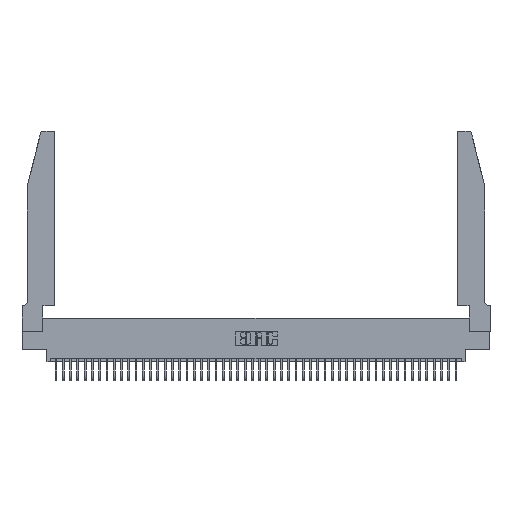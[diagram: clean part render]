
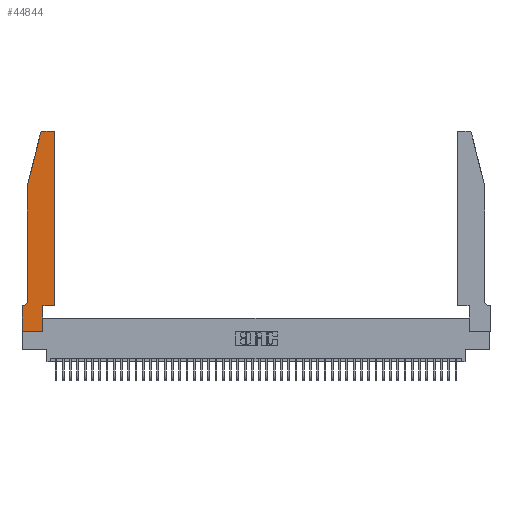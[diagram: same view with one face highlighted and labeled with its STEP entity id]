
A CAD part, top view. The second image highlights one B-rep face of the part: STEP entity #44844.
In plain terms, the highlighted planar face has unit normal (0, 0, 1).
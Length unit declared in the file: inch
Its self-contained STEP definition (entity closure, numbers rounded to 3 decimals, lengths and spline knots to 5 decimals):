
#1173 = CARTESIAN_POINT ( 'NONE',  ( 0.284, 2.75, 0.37 ) ) ;
#1705 = DIRECTION ( 'NONE',  ( 0., 0., -1. ) ) ;
#1728 = LINE ( 'NONE', #22792, #20487 ) ;
#2215 = DIRECTION ( 'NONE',  ( 0., 0., 1. ) ) ;
#2640 = ORIENTED_EDGE ( 'NONE', *, *, #30692, .T. ) ;
#3220 = DIRECTION ( 'NONE',  ( 0., 0., 1. ) ) ;
#3641 = AXIS2_PLACEMENT_3D ( 'NONE', #38031, #17236, #41556 ) ;
#4060 = ORIENTED_EDGE ( 'NONE', *, *, #23401, .T. ) ;
#4493 = ORIENTED_EDGE ( 'NONE', *, *, #15416, .T. ) ;
#4783 = CARTESIAN_POINT ( 'NONE',  ( 0.4205, 2.75, 0.37 ) ) ;
#5003 = VERTEX_POINT ( 'NONE', #37619 ) ;
#5460 = ORIENTED_EDGE ( 'NONE', *, *, #25876, .T. ) ;
#5517 = VERTEX_POINT ( 'NONE', #40341 ) ;
#5669 = ORIENTED_EDGE ( 'NONE', *, *, #30550, .T. ) ;
#6567 = DIRECTION ( 'NONE',  ( 0., -1., 0. ) ) ;
#6885 = EDGE_CURVE ( 'NONE', #39314, #39342, #33045, .T. ) ;
#7186 = CARTESIAN_POINT ( 'NONE',  ( 0.4505, 0.35, 0.37 ) ) ;
#7637 = VECTOR ( 'NONE', #6567, 39.37008 ) ;
#7947 = CARTESIAN_POINT ( 'NONE',  ( 0.0755, 0.35, 0.37 ) ) ;
#8311 = CIRCLE ( 'NONE', #44895, 0.03 ) ;
#8340 = VECTOR ( 'NONE', #38804, 39.37008 ) ;
#8362 = EDGE_CURVE ( 'NONE', #38802, #43409, #1728, .T. ) ;
#8693 = DIRECTION ( 'NONE',  ( -0.239, -0.971, 0. ) ) ;
#9033 = CARTESIAN_POINT ( 'NONE',  ( 0., 0.35, 0.37 ) ) ;
#9128 = VERTEX_POINT ( 'NONE', #20470 ) ;
#10287 = CIRCLE ( 'NONE', #3641, 0.03 ) ;
#10928 = CARTESIAN_POINT ( 'NONE',  ( 0.25487, 2.72718, 0.37 ) ) ;
#13617 = AXIS2_PLACEMENT_3D ( 'NONE', #33557, #2215, #26706 ) ;
#14084 = DIRECTION ( 'NONE',  ( 0., 1., 0. ) ) ;
#14966 = CARTESIAN_POINT ( 'NONE',  ( 0.0755, 2., 0.37 ) ) ;
#15416 = EDGE_CURVE ( 'NONE', #9128, #39314, #26887, .T. ) ;
#16180 = ORIENTED_EDGE ( 'NONE', *, *, #40834, .T. ) ;
#16627 = DIRECTION ( 'NONE',  ( -1., 0., 0. ) ) ;
#16882 = ORIENTED_EDGE ( 'NONE', *, *, #43784, .T. ) ;
#17236 = DIRECTION ( 'NONE',  ( 0., 0., 1. ) ) ;
#17279 = FACE_OUTER_BOUND ( 'NONE', #21320, .T. ) ;
#19246 = VECTOR ( 'NONE', #42854, 39.37008 ) ;
#20470 = CARTESIAN_POINT ( 'NONE',  ( 0.2865, 0.35, 0.37 ) ) ;
#20487 = VECTOR ( 'NONE', #8693, 39.37008 ) ;
#20929 = ORIENTED_EDGE ( 'NONE', *, *, #38671, .T. ) ;
#21320 = EDGE_LOOP ( 'NONE', ( #4060, #20929, #37957, #5460, #22367, #42710, #16882, #16180, #5669, #4493, #29392, #2640 ) ) ;
#21464 = LINE ( 'NONE', #7947, #19246 ) ;
#22047 = VECTOR ( 'NONE', #44120, 39.37008 ) ;
#22367 = ORIENTED_EDGE ( 'NONE', *, *, #32344, .T. ) ;
#22773 = CARTESIAN_POINT ( 'NONE',  ( 0.0055, 0.42, 0.37 ) ) ;
#22792 = CARTESIAN_POINT ( 'NONE',  ( 0.0755, 2., 0.37 ) ) ;
#23273 = PLANE ( 'NONE',  #13617 ) ;
#23401 = EDGE_CURVE ( 'NONE', #28050, #35162, #42786, .T. ) ;
#23751 = VECTOR ( 'NONE', #29623, 39.37008 ) ;
#24238 = CARTESIAN_POINT ( 'NONE',  ( 0.4205, 2.72, 0.37 ) ) ;
#25876 = EDGE_CURVE ( 'NONE', #43409, #5003, #31627, .T. ) ;
#26091 = CARTESIAN_POINT ( 'NONE',  ( 0.0755, 2., 0.37 ) ) ;
#26190 = DIRECTION ( 'NONE',  ( -1., 0., 0. ) ) ;
#26706 = DIRECTION ( 'NONE',  ( 1., 0., 0. ) ) ;
#26887 = LINE ( 'NONE', #28304, #8340 ) ;
#27705 = DIRECTION ( 'NONE',  ( 1., 0., 0. ) ) ;
#28050 = VERTEX_POINT ( 'NONE', #4783 ) ;
#28246 = CARTESIAN_POINT ( 'NONE',  ( 0.4505, 2.72, 0.37 ) ) ;
#28304 = CARTESIAN_POINT ( 'NONE',  ( 0.4505, 0.35, 0.37 ) ) ;
#29392 = ORIENTED_EDGE ( 'NONE', *, *, #6885, .T. ) ;
#29623 = DIRECTION ( 'NONE',  ( 1., 0., 0. ) ) ;
#30550 = EDGE_CURVE ( 'NONE', #5517, #9128, #40528, .T. ) ;
#30692 = EDGE_CURVE ( 'NONE', #39342, #28050, #8311, .T. ) ;
#31295 = AXIS2_PLACEMENT_3D ( 'NONE', #22773, #1705, #26190 ) ;
#31627 = LINE ( 'NONE', #26091, #39801 ) ;
#32344 = EDGE_CURVE ( 'NONE', #5003, #33185, #34839, .T. ) ;
#32946 = LINE ( 'NONE', #43610, #23751 ) ;
#33045 = LINE ( 'NONE', #38526, #42332 ) ;
#33185 = VERTEX_POINT ( 'NONE', #38495 ) ;
#33557 = CARTESIAN_POINT ( 'NONE',  ( 0., 0.35, 0.37 ) ) ;
#34577 = VECTOR ( 'NONE', #16627, 39.37008 ) ;
#34839 = CIRCLE ( 'NONE', #31295, 0.07 ) ;
#35162 = VERTEX_POINT ( 'NONE', #1173 ) ;
#35440 = LINE ( 'NONE', #44792, #7637 ) ;
#36590 = DIRECTION ( 'NONE',  ( 0., -1., 0. ) ) ;
#37155 = CARTESIAN_POINT ( 'NONE',  ( 0.2865, 0.35, 0.37 ) ) ;
#37302 = VERTEX_POINT ( 'NONE', #9033 ) ;
#37619 = CARTESIAN_POINT ( 'NONE',  ( 0.0755, 0.42, 0.37 ) ) ;
#37620 = VERTEX_POINT ( 'NONE', #42075 ) ;
#37957 = ORIENTED_EDGE ( 'NONE', *, *, #8362, .T. ) ;
#38031 = CARTESIAN_POINT ( 'NONE',  ( 0.284, 2.72, 0.37 ) ) ;
#38495 = CARTESIAN_POINT ( 'NONE',  ( 0.0055, 0.35, 0.37 ) ) ;
#38526 = CARTESIAN_POINT ( 'NONE',  ( 0.4505, 0.35, 0.37 ) ) ;
#38671 = EDGE_CURVE ( 'NONE', #35162, #38802, #10287, .T. ) ;
#38802 = VERTEX_POINT ( 'NONE', #10928 ) ;
#38804 = DIRECTION ( 'NONE',  ( 1., 0., 0. ) ) ;
#39314 = VERTEX_POINT ( 'NONE', #7186 ) ;
#39342 = VERTEX_POINT ( 'NONE', #28246 ) ;
#39801 = VECTOR ( 'NONE', #36590, 39.37008 ) ;
#40341 = CARTESIAN_POINT ( 'NONE',  ( 0.2865, 0., 0.37 ) ) ;
#40528 = LINE ( 'NONE', #37155, #22047 ) ;
#40834 = EDGE_CURVE ( 'NONE', #37620, #5517, #32946, .T. ) ;
#40942 = CARTESIAN_POINT ( 'NONE',  ( 0.2605, 2.75, 0.37 ) ) ;
#41556 = DIRECTION ( 'NONE',  ( 1., 0., 0. ) ) ;
#42075 = CARTESIAN_POINT ( 'NONE',  ( 0., 0., 0.37 ) ) ;
#42169 = EDGE_CURVE ( 'NONE', #33185, #37302, #21464, .T. ) ;
#42332 = VECTOR ( 'NONE', #14084, 39.37008 ) ;
#42710 = ORIENTED_EDGE ( 'NONE', *, *, #42169, .T. ) ;
#42786 = LINE ( 'NONE', #40942, #34577 ) ;
#42854 = DIRECTION ( 'NONE',  ( -1., 0., 0. ) ) ;
#43409 = VERTEX_POINT ( 'NONE', #14966 ) ;
#43610 = CARTESIAN_POINT ( 'NONE',  ( 0., 0., 0.37 ) ) ;
#43784 = EDGE_CURVE ( 'NONE', #37302, #37620, #35440, .T. ) ;
#44120 = DIRECTION ( 'NONE',  ( 0., 1., 0. ) ) ;
#44792 = CARTESIAN_POINT ( 'NONE',  ( 0., 0., 0.37 ) ) ;
#44844 = ADVANCED_FACE ( 'NONE', ( #17279 ), #23273, .T. ) ;
#44895 = AXIS2_PLACEMENT_3D ( 'NONE', #24238, #3220, #27705 ) ;
